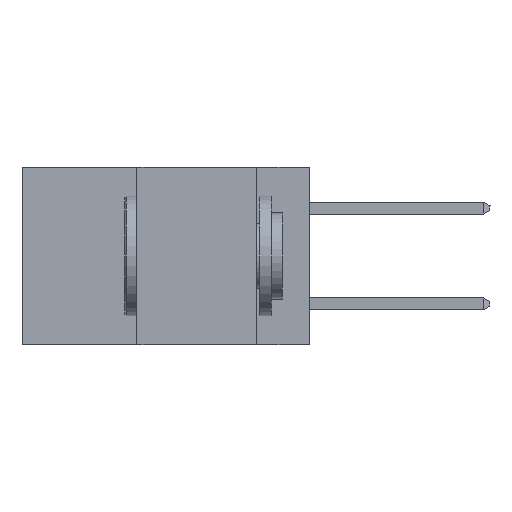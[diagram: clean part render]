
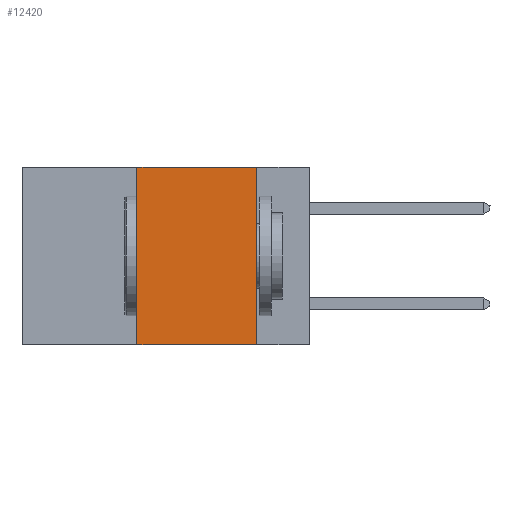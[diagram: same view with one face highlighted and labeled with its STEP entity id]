
A CAD part, left-side view. The second image highlights one B-rep face of the part: STEP entity #12420.
In plain terms, the highlighted planar face has unit normal (-1, 0, 0).
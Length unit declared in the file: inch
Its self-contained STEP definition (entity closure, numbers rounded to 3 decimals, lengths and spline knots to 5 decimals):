
#58 = DIRECTION ( 'NONE',  ( 0., 0., 1. ) ) ;
#209 = CARTESIAN_POINT ( 'NONE',  ( 0., 0.11, 0. ) ) ;
#271 = EDGE_CURVE ( 'NONE', #1115, #3322, #11225, .T. ) ;
#1115 = VERTEX_POINT ( 'NONE', #9180 ) ;
#1298 = CARTESIAN_POINT ( 'NONE',  ( 0., 0.6, 0. ) ) ;
#1461 = ORIENTED_EDGE ( 'NONE', *, *, #5315, .F. ) ;
#1512 = VECTOR ( 'NONE', #9860, 39.37008 ) ;
#1684 = EDGE_CURVE ( 'NONE', #3442, #3322, #13472, .T. ) ;
#1990 = DIRECTION ( 'NONE',  ( 0., -1., 0. ) ) ;
#2047 = VERTEX_POINT ( 'NONE', #9279 ) ;
#2400 = DIRECTION ( 'NONE',  ( 0., 0., -1. ) ) ;
#2598 = EDGE_LOOP ( 'NONE', ( #3672, #1461, #6953, #7114 ) ) ;
#3004 = LINE ( 'NONE', #6338, #9874 ) ;
#3322 = VERTEX_POINT ( 'NONE', #4397 ) ;
#3339 = DIRECTION ( 'NONE',  ( 0., 0., -1. ) ) ;
#3442 = VERTEX_POINT ( 'NONE', #10046 ) ;
#3672 = ORIENTED_EDGE ( 'NONE', *, *, #1684, .F. ) ;
#4397 = CARTESIAN_POINT ( 'NONE',  ( 0., 0.11, -0.37 ) ) ;
#4612 = CARTESIAN_POINT ( 'NONE',  ( 0., 0.6, 0. ) ) ;
#5220 = CARTESIAN_POINT ( 'NONE',  ( 0., 0.6, -0.37 ) ) ;
#5315 = EDGE_CURVE ( 'NONE', #2047, #3442, #10570, .T. ) ;
#6338 = CARTESIAN_POINT ( 'NONE',  ( 0., 0.36, 0. ) ) ;
#6953 = ORIENTED_EDGE ( 'NONE', *, *, #12476, .F. ) ;
#7052 = PLANE ( 'NONE',  #9567 ) ;
#7114 = ORIENTED_EDGE ( 'NONE', *, *, #271, .T. ) ;
#9180 = CARTESIAN_POINT ( 'NONE',  ( 0., 0.36, -0.37 ) ) ;
#9279 = CARTESIAN_POINT ( 'NONE',  ( 0., 0.36, 0. ) ) ;
#9391 = FACE_OUTER_BOUND ( 'NONE', #2598, .T. ) ;
#9567 = AXIS2_PLACEMENT_3D ( 'NONE', #1298, #9710, #2400 ) ;
#9710 = DIRECTION ( 'NONE',  ( 1., 0., 0. ) ) ;
#9860 = DIRECTION ( 'NONE',  ( 0., -1., 0. ) ) ;
#9874 = VECTOR ( 'NONE', #58, 39.37008 ) ;
#9990 = VECTOR ( 'NONE', #3339, 39.37008 ) ;
#10046 = CARTESIAN_POINT ( 'NONE',  ( 0., 0.11, 0. ) ) ;
#10570 = LINE ( 'NONE', #4612, #1512 ) ;
#11225 = LINE ( 'NONE', #5220, #11705 ) ;
#11705 = VECTOR ( 'NONE', #1990, 39.37008 ) ;
#12420 = ADVANCED_FACE ( 'NONE', ( #9391 ), #7052, .F. ) ;
#12476 = EDGE_CURVE ( 'NONE', #1115, #2047, #3004, .T. ) ;
#13472 = LINE ( 'NONE', #209, #9990 ) ;
